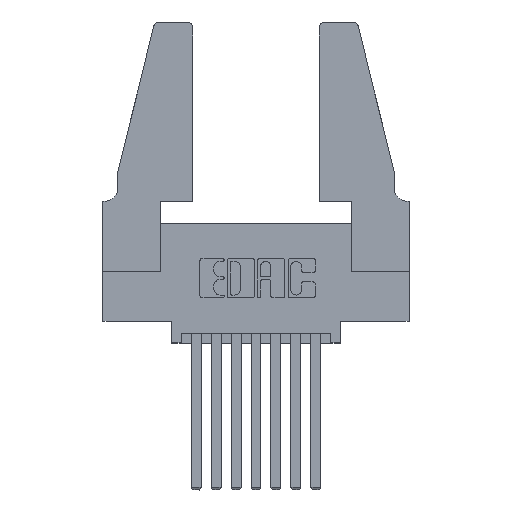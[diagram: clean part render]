
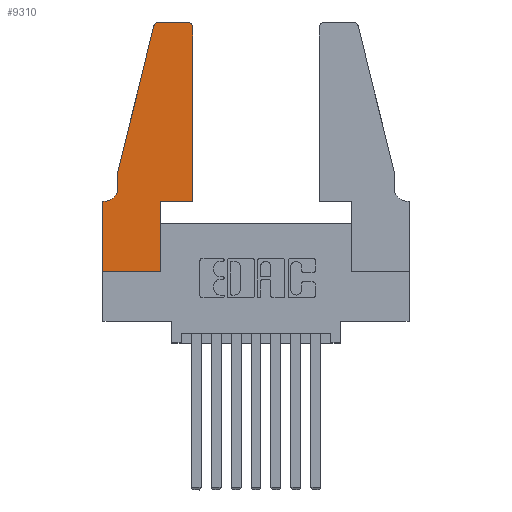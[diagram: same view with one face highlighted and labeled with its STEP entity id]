
A CAD part, top view. The second image highlights one B-rep face of the part: STEP entity #9310.
In plain terms, the highlighted planar face has unit normal (0, 0, 1).
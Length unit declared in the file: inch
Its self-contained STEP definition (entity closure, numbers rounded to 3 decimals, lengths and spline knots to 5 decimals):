
#214 = ORIENTED_EDGE ( 'NONE', *, *, #9045, .T. ) ;
#248 = FACE_OUTER_BOUND ( 'NONE', #10358, .T. ) ;
#367 = DIRECTION ( 'NONE',  ( 1., 0., 0. ) ) ;
#419 = DIRECTION ( 'NONE',  ( -1., 0., 0. ) ) ;
#437 = DIRECTION ( 'NONE',  ( 0., 1., 0. ) ) ;
#598 = LINE ( 'NONE', #6201, #3854 ) ;
#820 = AXIS2_PLACEMENT_3D ( 'NONE', #6065, #11915, #367 ) ;
#834 = EDGE_CURVE ( 'NONE', #11920, #7585, #10219, .T. ) ;
#865 = VECTOR ( 'NONE', #2061, 39.37008 ) ;
#986 = VERTEX_POINT ( 'NONE', #11024 ) ;
#1023 = ORIENTED_EDGE ( 'NONE', *, *, #8240, .T. ) ;
#1335 = ORIENTED_EDGE ( 'NONE', *, *, #7118, .T. ) ;
#1429 = AXIS2_PLACEMENT_3D ( 'NONE', #6941, #5975, #5012 ) ;
#1460 = EDGE_CURVE ( 'NONE', #986, #11920, #2142, .T. ) ;
#1468 = VERTEX_POINT ( 'NONE', #7321 ) ;
#1513 = DIRECTION ( 'NONE',  ( 0., -1., 0. ) ) ;
#1543 = DIRECTION ( 'NONE',  ( 1., 0., 0. ) ) ;
#1751 = LINE ( 'NONE', #4798, #10233 ) ;
#1910 = EDGE_CURVE ( 'NONE', #4391, #6008, #3330, .T. ) ;
#1943 = CARTESIAN_POINT ( 'NONE',  ( 0.25487, 1.22718, 0.37 ) ) ;
#2061 = DIRECTION ( 'NONE',  ( 0., 1., 0. ) ) ;
#2142 = LINE ( 'NONE', #12177, #12305 ) ;
#2145 = LINE ( 'NONE', #5124, #3665 ) ;
#2204 = CARTESIAN_POINT ( 'NONE',  ( 0.0755, 0.42, 0.37 ) ) ;
#2582 = CARTESIAN_POINT ( 'NONE',  ( 0., 0., 0.37 ) ) ;
#2865 = VERTEX_POINT ( 'NONE', #10540 ) ;
#3092 = CIRCLE ( 'NONE', #820, 0.03 ) ;
#3204 = AXIS2_PLACEMENT_3D ( 'NONE', #4276, #3219, #1543 ) ;
#3219 = DIRECTION ( 'NONE',  ( 0., 0., 1. ) ) ;
#3304 = ORIENTED_EDGE ( 'NONE', *, *, #1910, .T. ) ;
#3322 = CARTESIAN_POINT ( 'NONE',  ( 0.2865, 0., 0.37 ) ) ;
#3330 = CIRCLE ( 'NONE', #1429, 0.07 ) ;
#3399 = CARTESIAN_POINT ( 'NONE',  ( 0.0755, 0.5, 0.37 ) ) ;
#3664 = DIRECTION ( 'NONE',  ( 0., 0., 1. ) ) ;
#3665 = VECTOR ( 'NONE', #11760, 39.37008 ) ;
#3688 = DIRECTION ( 'NONE',  ( 1., 0., 0. ) ) ;
#3701 = DIRECTION ( 'NONE',  ( 0., -1., 0. ) ) ;
#3854 = VECTOR ( 'NONE', #419, 39.37008 ) ;
#4276 = CARTESIAN_POINT ( 'NONE',  ( 0., 0.35, 0.37 ) ) ;
#4391 = VERTEX_POINT ( 'NONE', #2204 ) ;
#4409 = DIRECTION ( 'NONE',  ( 1., 0., 0. ) ) ;
#4709 = VERTEX_POINT ( 'NONE', #10637 ) ;
#4798 = CARTESIAN_POINT ( 'NONE',  ( 0.2605, 1.25, 0.37 ) ) ;
#4877 = DIRECTION ( 'NONE',  ( -1., 0., 0. ) ) ;
#5012 = DIRECTION ( 'NONE',  ( -1., 0., 0. ) ) ;
#5124 = CARTESIAN_POINT ( 'NONE',  ( 0.0755, 0.5, 0.37 ) ) ;
#5231 = ORIENTED_EDGE ( 'NONE', *, *, #8964, .T. ) ;
#5316 = PLANE ( 'NONE',  #3204 ) ;
#5451 = CARTESIAN_POINT ( 'NONE',  ( 0., 0., 0.37 ) ) ;
#5696 = EDGE_CURVE ( 'NONE', #4709, #8581, #3092, .T. ) ;
#5779 = VECTOR ( 'NONE', #6234, 39.37008 ) ;
#5975 = DIRECTION ( 'NONE',  ( 0., 0., -1. ) ) ;
#6008 = VERTEX_POINT ( 'NONE', #10370 ) ;
#6065 = CARTESIAN_POINT ( 'NONE',  ( 0.284, 1.22, 0.37 ) ) ;
#6201 = CARTESIAN_POINT ( 'NONE',  ( 0.0755, 0.35, 0.37 ) ) ;
#6234 = DIRECTION ( 'NONE',  ( 1., 0., 0. ) ) ;
#6389 = LINE ( 'NONE', #10369, #11443 ) ;
#6777 = ORIENTED_EDGE ( 'NONE', *, *, #1460, .T. ) ;
#6808 = CARTESIAN_POINT ( 'NONE',  ( 0.4505, 0.35, 0.37 ) ) ;
#6941 = CARTESIAN_POINT ( 'NONE',  ( 0.0055, 0.42, 0.37 ) ) ;
#6944 = EDGE_CURVE ( 'NONE', #10315, #4391, #10265, .T. ) ;
#7118 = EDGE_CURVE ( 'NONE', #11501, #7935, #11457, .T. ) ;
#7321 = CARTESIAN_POINT ( 'NONE',  ( 0.4505, 0.35, 0.37 ) ) ;
#7585 = VERTEX_POINT ( 'NONE', #3322 ) ;
#7829 = AXIS2_PLACEMENT_3D ( 'NONE', #9358, #3664, #4409 ) ;
#7887 = EDGE_CURVE ( 'NONE', #7585, #2865, #8343, .T. ) ;
#7935 = VERTEX_POINT ( 'NONE', #12180 ) ;
#8048 = ORIENTED_EDGE ( 'NONE', *, *, #6944, .T. ) ;
#8061 = EDGE_CURVE ( 'NONE', #2865, #1468, #6389, .T. ) ;
#8099 = CARTESIAN_POINT ( 'NONE',  ( 0.2865, 0.35, 0.37 ) ) ;
#8158 = LINE ( 'NONE', #6808, #865 ) ;
#8182 = VECTOR ( 'NONE', #437, 39.37008 ) ;
#8240 = EDGE_CURVE ( 'NONE', #6008, #986, #598, .T. ) ;
#8343 = LINE ( 'NONE', #8099, #8182 ) ;
#8495 = VECTOR ( 'NONE', #1513, 39.37008 ) ;
#8581 = VERTEX_POINT ( 'NONE', #1943 ) ;
#8964 = EDGE_CURVE ( 'NONE', #7935, #4709, #1751, .T. ) ;
#9045 = EDGE_CURVE ( 'NONE', #1468, #11501, #8158, .T. ) ;
#9310 = ADVANCED_FACE ( 'NONE', ( #248 ), #5316, .T. ) ;
#9358 = CARTESIAN_POINT ( 'NONE',  ( 0.4205, 1.22, 0.37 ) ) ;
#9615 = ORIENTED_EDGE ( 'NONE', *, *, #10093, .T. ) ;
#9743 = ORIENTED_EDGE ( 'NONE', *, *, #7887, .T. ) ;
#10093 = EDGE_CURVE ( 'NONE', #8581, #10315, #2145, .T. ) ;
#10219 = LINE ( 'NONE', #5451, #5779 ) ;
#10233 = VECTOR ( 'NONE', #4877, 39.37008 ) ;
#10265 = LINE ( 'NONE', #10936, #8495 ) ;
#10315 = VERTEX_POINT ( 'NONE', #3399 ) ;
#10358 = EDGE_LOOP ( 'NONE', ( #5231, #11919, #9615, #8048, #3304, #1023, #6777, #11675, #9743, #11624, #214, #1335 ) ) ;
#10369 = CARTESIAN_POINT ( 'NONE',  ( 0.4505, 0.35, 0.37 ) ) ;
#10370 = CARTESIAN_POINT ( 'NONE',  ( 0.0055, 0.35, 0.37 ) ) ;
#10540 = CARTESIAN_POINT ( 'NONE',  ( 0.2865, 0.35, 0.37 ) ) ;
#10637 = CARTESIAN_POINT ( 'NONE',  ( 0.284, 1.25, 0.37 ) ) ;
#10935 = CARTESIAN_POINT ( 'NONE',  ( 0.4505, 1.22, 0.37 ) ) ;
#10936 = CARTESIAN_POINT ( 'NONE',  ( 0.0755, 0.5, 0.37 ) ) ;
#11024 = CARTESIAN_POINT ( 'NONE',  ( 0., 0.35, 0.37 ) ) ;
#11443 = VECTOR ( 'NONE', #3688, 39.37008 ) ;
#11457 = CIRCLE ( 'NONE', #7829, 0.03 ) ;
#11501 = VERTEX_POINT ( 'NONE', #10935 ) ;
#11624 = ORIENTED_EDGE ( 'NONE', *, *, #8061, .T. ) ;
#11675 = ORIENTED_EDGE ( 'NONE', *, *, #834, .T. ) ;
#11760 = DIRECTION ( 'NONE',  ( -0.239, -0.971, 0. ) ) ;
#11915 = DIRECTION ( 'NONE',  ( 0., 0., 1. ) ) ;
#11919 = ORIENTED_EDGE ( 'NONE', *, *, #5696, .T. ) ;
#11920 = VERTEX_POINT ( 'NONE', #2582 ) ;
#12177 = CARTESIAN_POINT ( 'NONE',  ( 0., 0., 0.37 ) ) ;
#12180 = CARTESIAN_POINT ( 'NONE',  ( 0.4205, 1.25, 0.37 ) ) ;
#12305 = VECTOR ( 'NONE', #3701, 39.37008 ) ;
